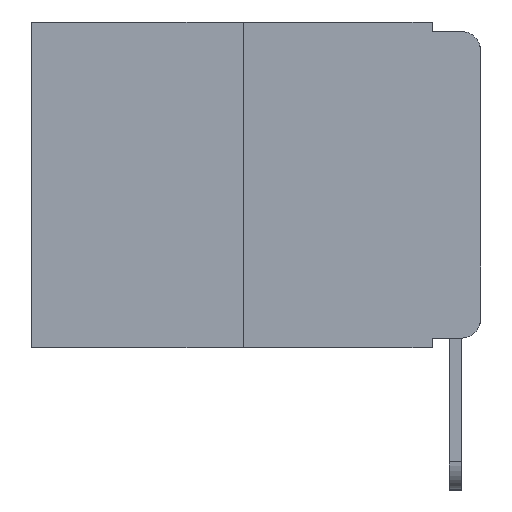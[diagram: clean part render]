
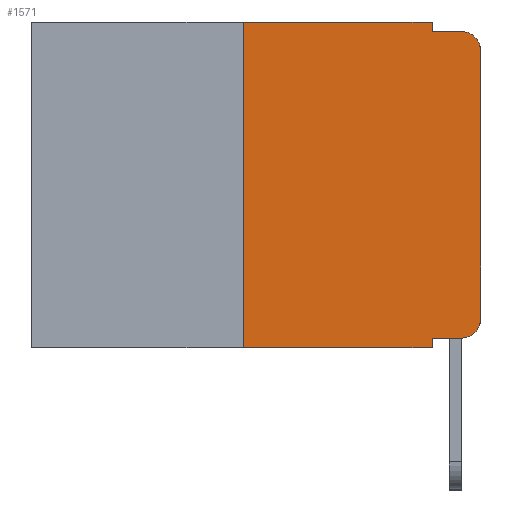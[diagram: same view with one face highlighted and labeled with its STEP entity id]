
A CAD part, left-side view. The second image highlights one B-rep face of the part: STEP entity #1571.
In plain terms, the highlighted planar face has unit normal (-1, 0, 0).
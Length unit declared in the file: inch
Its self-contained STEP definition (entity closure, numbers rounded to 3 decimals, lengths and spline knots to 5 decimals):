
#69 = LINE ( 'NONE', #7064, #8418 ) ;
#251 = AXIS2_PLACEMENT_3D ( 'NONE', #5100, #11346, #5138 ) ;
#350 = CARTESIAN_POINT ( 'NONE',  ( 0., 0.051, -0.333 ) ) ;
#396 = VERTEX_POINT ( 'NONE', #5268 ) ;
#500 = CARTESIAN_POINT ( 'NONE',  ( 0., 0.051, -0.343 ) ) ;
#505 = EDGE_CURVE ( 'NONE', #7575, #12424, #7018, .T. ) ;
#818 = CARTESIAN_POINT ( 'NONE',  ( 0., 0.051, 0. ) ) ;
#1130 = DIRECTION ( 'NONE',  ( -1., 0., 0. ) ) ;
#1178 = CARTESIAN_POINT ( 'NONE',  ( 0., 0., 0. ) ) ;
#1222 = VECTOR ( 'NONE', #7305, 39.37008 ) ;
#1294 = LINE ( 'NONE', #4783, #12795 ) ;
#1568 = LINE ( 'NONE', #13050, #7251 ) ;
#1571 = ADVANCED_FACE ( 'NONE', ( #12754 ), #11304, .F. ) ;
#1766 = DIRECTION ( 'NONE',  ( 0., -1., 0. ) ) ;
#1890 = CARTESIAN_POINT ( 'NONE',  ( 0., 0.02, -0.01 ) ) ;
#2067 = CARTESIAN_POINT ( 'NONE',  ( 0., 0.051, -0.333 ) ) ;
#2151 = ORIENTED_EDGE ( 'NONE', *, *, #8042, .F. ) ;
#2217 = EDGE_CURVE ( 'NONE', #4653, #11880, #69, .T. ) ;
#2249 = CARTESIAN_POINT ( 'NONE',  ( 0., 0.051, 0. ) ) ;
#2335 = AXIS2_PLACEMENT_3D ( 'NONE', #9615, #3362, #10653 ) ;
#2776 = DIRECTION ( 'NONE',  ( 0., -1., 0. ) ) ;
#2861 = LINE ( 'NONE', #12683, #5374 ) ;
#3307 = AXIS2_PLACEMENT_3D ( 'NONE', #7579, #1130, #8604 ) ;
#3362 = DIRECTION ( 'NONE',  ( -1., 0., 0. ) ) ;
#3611 = LINE ( 'NONE', #1178, #8823 ) ;
#3734 = VECTOR ( 'NONE', #8373, 39.37008 ) ;
#4487 = DIRECTION ( 'NONE',  ( 0., 0., 1. ) ) ;
#4653 = VERTEX_POINT ( 'NONE', #9059 ) ;
#4668 = EDGE_CURVE ( 'NONE', #12000, #9917, #1568, .T. ) ;
#4783 = CARTESIAN_POINT ( 'NONE',  ( 0., 0.051, 0. ) ) ;
#5009 = ORIENTED_EDGE ( 'NONE', *, *, #10137, .F. ) ;
#5100 = CARTESIAN_POINT ( 'NONE',  ( 0., 0.473, 0. ) ) ;
#5138 = DIRECTION ( 'NONE',  ( 0., 0., -1. ) ) ;
#5268 = CARTESIAN_POINT ( 'NONE',  ( 0., 0., -0.03 ) ) ;
#5342 = ORIENTED_EDGE ( 'NONE', *, *, #12177, .F. ) ;
#5374 = VECTOR ( 'NONE', #6564, 39.37008 ) ;
#5452 = CARTESIAN_POINT ( 'NONE',  ( 0., 0.051, -0.01 ) ) ;
#5550 = LINE ( 'NONE', #2067, #3734 ) ;
#5996 = ORIENTED_EDGE ( 'NONE', *, *, #12844, .F. ) ;
#6260 = CARTESIAN_POINT ( 'NONE',  ( 0., 0.25, 0. ) ) ;
#6327 = ORIENTED_EDGE ( 'NONE', *, *, #505, .T. ) ;
#6500 = DIRECTION ( 'NONE',  ( 0., -1., 0. ) ) ;
#6564 = DIRECTION ( 'NONE',  ( 0., 0., 1. ) ) ;
#6681 = EDGE_CURVE ( 'NONE', #12424, #396, #3611, .T. ) ;
#6808 = EDGE_LOOP ( 'NONE', ( #9878, #7424, #2151, #5009, #7757, #5342, #8406, #5996, #8721, #6327 ) ) ;
#7018 = CIRCLE ( 'NONE', #2335, 0.02 ) ;
#7064 = CARTESIAN_POINT ( 'NONE',  ( 0., 0.473, -0.343 ) ) ;
#7251 = VECTOR ( 'NONE', #2776, 39.37008 ) ;
#7305 = DIRECTION ( 'NONE',  ( 0., 0., -1. ) ) ;
#7350 = EDGE_CURVE ( 'NONE', #396, #7785, #9633, .T. ) ;
#7424 = ORIENTED_EDGE ( 'NONE', *, *, #7350, .T. ) ;
#7575 = VERTEX_POINT ( 'NONE', #8968 ) ;
#7579 = CARTESIAN_POINT ( 'NONE',  ( 0., 0.02, -0.03 ) ) ;
#7757 = ORIENTED_EDGE ( 'NONE', *, *, #4668, .F. ) ;
#7785 = VERTEX_POINT ( 'NONE', #1890 ) ;
#8042 = EDGE_CURVE ( 'NONE', #11428, #7785, #11150, .T. ) ;
#8369 = CARTESIAN_POINT ( 'NONE',  ( 0., 0.051, -0.01 ) ) ;
#8373 = DIRECTION ( 'NONE',  ( 0., -1., 0. ) ) ;
#8376 = VECTOR ( 'NONE', #6500, 39.37008 ) ;
#8406 = ORIENTED_EDGE ( 'NONE', *, *, #2217, .T. ) ;
#8418 = VECTOR ( 'NONE', #1766, 39.37008 ) ;
#8604 = DIRECTION ( 'NONE',  ( 0., 0., -1. ) ) ;
#8721 = ORIENTED_EDGE ( 'NONE', *, *, #13499, .T. ) ;
#8823 = VECTOR ( 'NONE', #4487, 39.37008 ) ;
#8952 = DIRECTION ( 'NONE',  ( 0., 0., -1. ) ) ;
#8968 = CARTESIAN_POINT ( 'NONE',  ( 0., 0.02, -0.333 ) ) ;
#9059 = CARTESIAN_POINT ( 'NONE',  ( 0., 0.25, -0.343 ) ) ;
#9615 = CARTESIAN_POINT ( 'NONE',  ( 0., 0.02, -0.313 ) ) ;
#9633 = CIRCLE ( 'NONE', #3307, 0.02 ) ;
#9728 = LINE ( 'NONE', #818, #1222 ) ;
#9878 = ORIENTED_EDGE ( 'NONE', *, *, #6681, .T. ) ;
#9917 = VERTEX_POINT ( 'NONE', #2249 ) ;
#10137 = EDGE_CURVE ( 'NONE', #9917, #11428, #1294, .T. ) ;
#10653 = DIRECTION ( 'NONE',  ( 0., 0., -1. ) ) ;
#11150 = LINE ( 'NONE', #5452, #8376 ) ;
#11304 = PLANE ( 'NONE',  #251 ) ;
#11346 = DIRECTION ( 'NONE',  ( 1., 0., 0. ) ) ;
#11428 = VERTEX_POINT ( 'NONE', #8369 ) ;
#11804 = VERTEX_POINT ( 'NONE', #350 ) ;
#11880 = VERTEX_POINT ( 'NONE', #500 ) ;
#12000 = VERTEX_POINT ( 'NONE', #6260 ) ;
#12177 = EDGE_CURVE ( 'NONE', #4653, #12000, #2861, .T. ) ;
#12424 = VERTEX_POINT ( 'NONE', #13644 ) ;
#12683 = CARTESIAN_POINT ( 'NONE',  ( 0., 0.25, 0. ) ) ;
#12754 = FACE_OUTER_BOUND ( 'NONE', #6808, .T. ) ;
#12795 = VECTOR ( 'NONE', #8952, 39.37008 ) ;
#12844 = EDGE_CURVE ( 'NONE', #11804, #11880, #9728, .T. ) ;
#13050 = CARTESIAN_POINT ( 'NONE',  ( 0., 0.473, 0. ) ) ;
#13499 = EDGE_CURVE ( 'NONE', #11804, #7575, #5550, .T. ) ;
#13644 = CARTESIAN_POINT ( 'NONE',  ( 0., 0., -0.313 ) ) ;
